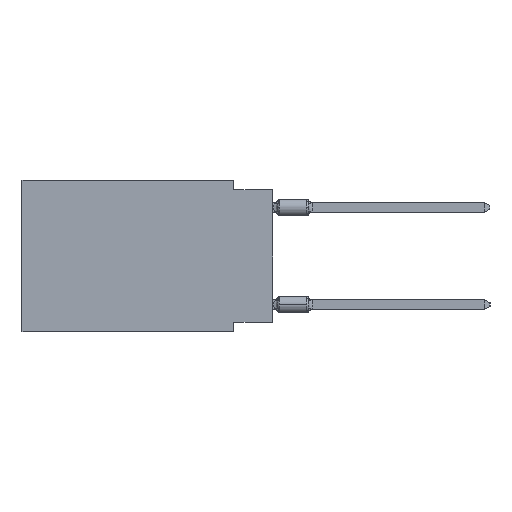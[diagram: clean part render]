
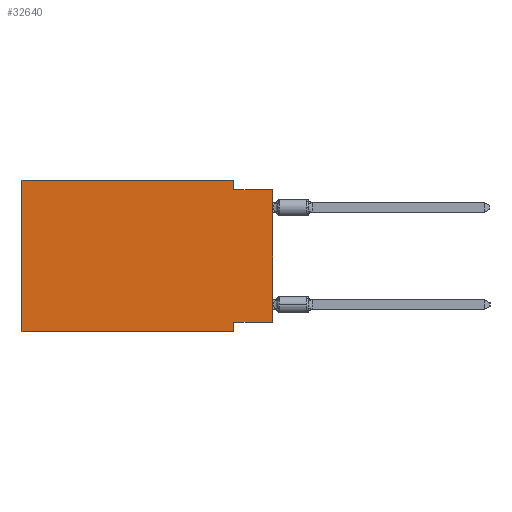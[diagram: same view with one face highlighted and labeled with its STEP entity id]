
A CAD part, left-side view. The second image highlights one B-rep face of the part: STEP entity #32640.
In plain terms, the highlighted planar face has unit normal (-1, 0, 0).
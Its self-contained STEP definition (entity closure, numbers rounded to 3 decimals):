
#669 = ORIENTED_EDGE ( 'NONE', *, *, #34902, .T. ) ;
#737 = VECTOR ( 'NONE', #5804, 1000. ) ;
#1743 = VECTOR ( 'NONE', #19529, 1000. ) ;
#1884 = LINE ( 'NONE', #7294, #1743 ) ;
#2121 = VECTOR ( 'NONE', #23426, 1000. ) ;
#4162 = EDGE_CURVE ( 'NONE', #24106, #27093, #7673, .T. ) ;
#4730 = EDGE_LOOP ( 'NONE', ( #30312, #10002, #27067, #26730, #24164, #669, #27571, #8976 ) ) ;
#5304 = DIRECTION ( 'NONE',  ( 0., 0., -1. ) ) ;
#5804 = DIRECTION ( 'NONE',  ( 0., -1., 0. ) ) ;
#6368 = VERTEX_POINT ( 'NONE', #21382 ) ;
#6784 = DIRECTION ( 'NONE',  ( 0., 0., -1. ) ) ;
#6890 = CARTESIAN_POINT ( 'NONE',  ( 0., 0., -9.271 ) ) ;
#7294 = CARTESIAN_POINT ( 'NONE',  ( 0., 0., 0. ) ) ;
#7374 = FACE_OUTER_BOUND ( 'NONE', #4730, .T. ) ;
#7673 = LINE ( 'NONE', #6890, #38137 ) ;
#8432 = VERTEX_POINT ( 'NONE', #20658 ) ;
#8976 = ORIENTED_EDGE ( 'NONE', *, *, #4162, .F. ) ;
#9164 = VECTOR ( 'NONE', #27709, 1000. ) ;
#9549 = CARTESIAN_POINT ( 'NONE',  ( 0., 0., -9.271 ) ) ;
#9889 = EDGE_CURVE ( 'NONE', #12161, #22771, #16802, .T. ) ;
#10002 = ORIENTED_EDGE ( 'NONE', *, *, #32553, .F. ) ;
#10174 = DIRECTION ( 'NONE',  ( 1., 0., 0. ) ) ;
#11117 = EDGE_CURVE ( 'NONE', #22771, #8432, #23830, .T. ) ;
#11522 = CARTESIAN_POINT ( 'NONE',  ( 0., 2.54, 0. ) ) ;
#11865 = DIRECTION ( 'NONE',  ( 0., 0., -1. ) ) ;
#12161 = VERTEX_POINT ( 'NONE', #30336 ) ;
#12611 = CARTESIAN_POINT ( 'NONE',  ( 0., 0., -0.635 ) ) ;
#14627 = EDGE_CURVE ( 'NONE', #8432, #6368, #36540, .T. ) ;
#14655 = VECTOR ( 'NONE', #11865, 1000. ) ;
#16722 = CARTESIAN_POINT ( 'NONE',  ( 0., 2.54, -9.271 ) ) ;
#16802 = LINE ( 'NONE', #17208, #25100 ) ;
#17208 = CARTESIAN_POINT ( 'NONE',  ( 0., 16.383, 0. ) ) ;
#17475 = LINE ( 'NONE', #26496, #14655 ) ;
#18027 = LINE ( 'NONE', #12611, #737 ) ;
#19409 = PLANE ( 'NONE',  #33983 ) ;
#19529 = DIRECTION ( 'NONE',  ( 0., 0., 1. ) ) ;
#20658 = CARTESIAN_POINT ( 'NONE',  ( 0., 2.54, 0. ) ) ;
#20841 = VERTEX_POINT ( 'NONE', #24105 ) ;
#21382 = CARTESIAN_POINT ( 'NONE',  ( 0., 2.54, -0.635 ) ) ;
#22771 = VERTEX_POINT ( 'NONE', #29028 ) ;
#23426 = DIRECTION ( 'NONE',  ( 0., -1., 0. ) ) ;
#23542 = CARTESIAN_POINT ( 'NONE',  ( 0., 0., -0.635 ) ) ;
#23830 = LINE ( 'NONE', #29247, #2121 ) ;
#24105 = CARTESIAN_POINT ( 'NONE',  ( 0., 2.54, -9.906 ) ) ;
#24106 = VERTEX_POINT ( 'NONE', #9549 ) ;
#24164 = ORIENTED_EDGE ( 'NONE', *, *, #9889, .F. ) ;
#25100 = VECTOR ( 'NONE', #29638, 1000. ) ;
#25360 = VECTOR ( 'NONE', #5304, 1000. ) ;
#25418 = CARTESIAN_POINT ( 'NONE',  ( 0., 16.383, 0. ) ) ;
#25785 = EDGE_CURVE ( 'NONE', #24106, #29703, #1884, .T. ) ;
#26496 = CARTESIAN_POINT ( 'NONE',  ( 0., 2.54, -9.906 ) ) ;
#26730 = ORIENTED_EDGE ( 'NONE', *, *, #11117, .F. ) ;
#27067 = ORIENTED_EDGE ( 'NONE', *, *, #14627, .F. ) ;
#27093 = VERTEX_POINT ( 'NONE', #16722 ) ;
#27571 = ORIENTED_EDGE ( 'NONE', *, *, #27674, .F. ) ;
#27674 = EDGE_CURVE ( 'NONE', #27093, #20841, #17475, .T. ) ;
#27709 = DIRECTION ( 'NONE',  ( 0., -1., 0. ) ) ;
#29028 = CARTESIAN_POINT ( 'NONE',  ( 0., 16.383, 0. ) ) ;
#29247 = CARTESIAN_POINT ( 'NONE',  ( 0., 16.383, 0. ) ) ;
#29638 = DIRECTION ( 'NONE',  ( 0., 0., 1. ) ) ;
#29703 = VERTEX_POINT ( 'NONE', #23542 ) ;
#30312 = ORIENTED_EDGE ( 'NONE', *, *, #25785, .T. ) ;
#30336 = CARTESIAN_POINT ( 'NONE',  ( 0., 16.383, -9.906 ) ) ;
#30504 = CARTESIAN_POINT ( 'NONE',  ( 0., 16.383, -9.906 ) ) ;
#31335 = DIRECTION ( 'NONE',  ( 0., 1., 0. ) ) ;
#32553 = EDGE_CURVE ( 'NONE', #6368, #29703, #18027, .T. ) ;
#32640 = ADVANCED_FACE ( 'NONE', ( #7374 ), #19409, .F. ) ;
#33698 = LINE ( 'NONE', #30504, #9164 ) ;
#33983 = AXIS2_PLACEMENT_3D ( 'NONE', #25418, #10174, #6784 ) ;
#34902 = EDGE_CURVE ( 'NONE', #12161, #20841, #33698, .T. ) ;
#36540 = LINE ( 'NONE', #11522, #25360 ) ;
#38137 = VECTOR ( 'NONE', #31335, 1000. ) ;
